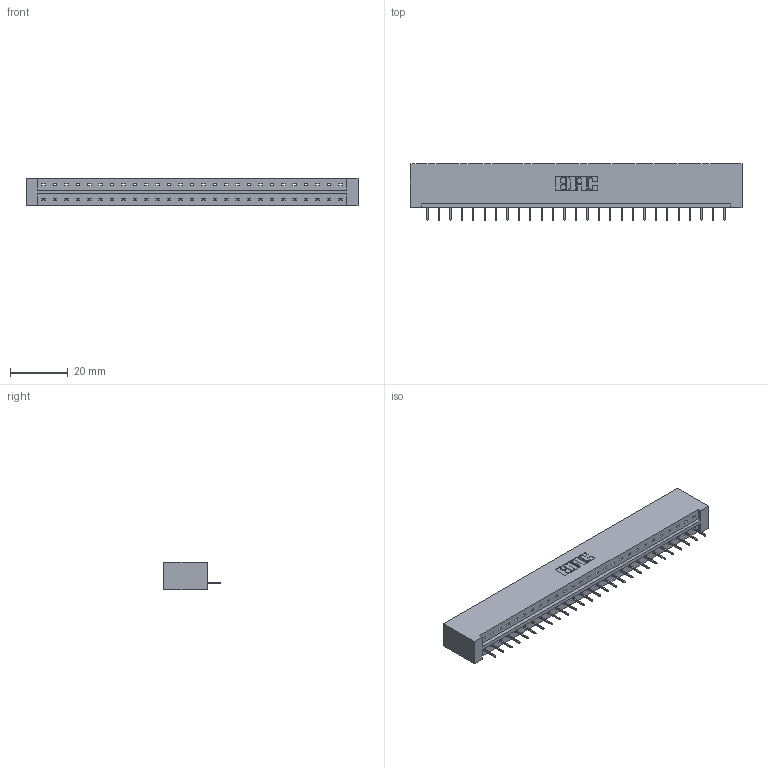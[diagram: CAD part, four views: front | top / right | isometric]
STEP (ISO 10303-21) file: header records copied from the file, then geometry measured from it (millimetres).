
FILE_DESCRIPTION (( 'STEP AP203' ), '1' );
FILE_NAME ('333-027-524-101.STEP', '2018-08-02T13:54:24', ( '' ), ( '' ), 'SwSTEP 2.0', 'SolidWorks 2016', '' );
FILE_SCHEMA (( 'CONFIG_CONTROL_DESIGN' ));
Length unit declared in the file: inch
Products named in the file (3): 333 Part_Lugless; 345-292-001_345-293-124; 333-027-524-101
Assembly tree (28 placements, depth 2):
  333-027-524-101
    333 Part_Lugless
    345-292-001_345-293-124  x27
Bounding box: 115.24 x 19.69 x 9.4 mm (x, y, z)
Volume: 11973.5 mm3; surface area: 12446.9 mm2
Topology: 28 solids, 28 shells, 1780 faces, 5147 edges, 3322 vertices
Faces by surface type: plane 1362, cylinder 418
Entity records: 18243 total; most frequent: CARTESIAN_POINT 3155, ORIENTED_EDGE 3118, DIRECTION 2685, EDGE_CURVE 1559, LINE 1443, VECTOR 1443, VERTEX_POINT 1034, AXIS2_PLACEMENT_3D 621
